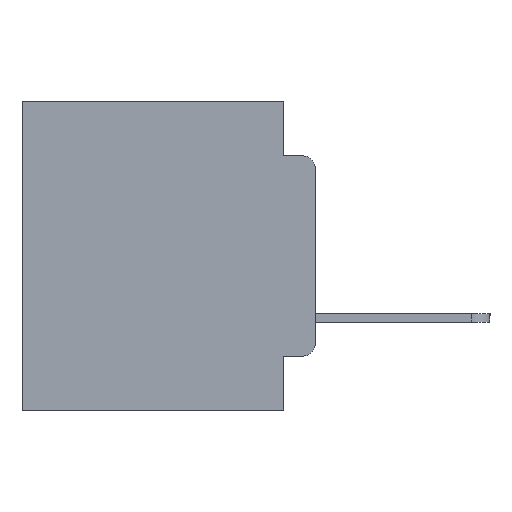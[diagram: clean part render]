
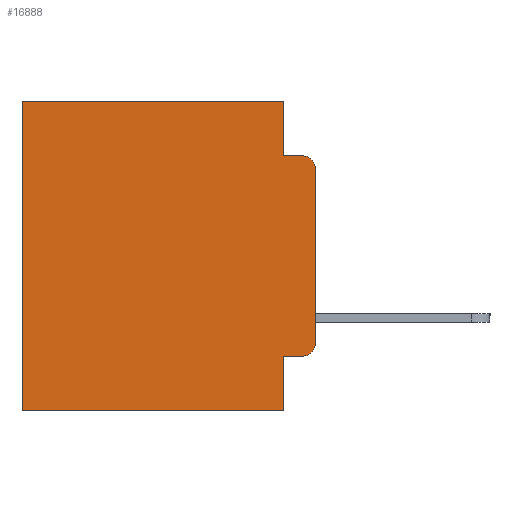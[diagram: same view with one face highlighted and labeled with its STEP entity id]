
A CAD part, left-side view. The second image highlights one B-rep face of the part: STEP entity #16888.
In plain terms, the highlighted planar face has unit normal (-1, 0, 0).
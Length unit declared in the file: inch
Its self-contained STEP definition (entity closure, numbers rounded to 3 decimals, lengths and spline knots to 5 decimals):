
#23 = CARTESIAN_POINT ( 'NONE',  ( 0.298, 0.02, -0.1085 ) ) ;
#478 = VERTEX_POINT ( 'NONE', #4145 ) ;
#646 = CARTESIAN_POINT ( 'NONE',  ( 0.298, 0.051, -0.4115 ) ) ;
#1078 = DIRECTION ( 'NONE',  ( 0., 1., 0. ) ) ;
#1101 = DIRECTION ( 'NONE',  ( 0., 0., -1. ) ) ;
#1195 = EDGE_CURVE ( 'NONE', #14143, #478, #6754, .T. ) ;
#1214 = DIRECTION ( 'NONE',  ( -1., 0., 0. ) ) ;
#1450 = ORIENTED_EDGE ( 'NONE', *, *, #19248, .T. ) ;
#1597 = VERTEX_POINT ( 'NONE', #25536 ) ;
#1932 = CARTESIAN_POINT ( 'NONE',  ( 0.298, 0.051, -0.0885 ) ) ;
#2301 = PLANE ( 'NONE',  #19564 ) ;
#2484 = ORIENTED_EDGE ( 'NONE', *, *, #11414, .F. ) ;
#2971 = CARTESIAN_POINT ( 'NONE',  ( 0.298, 0.051, 0. ) ) ;
#3621 = VECTOR ( 'NONE', #20673, 39.37008 ) ;
#3719 = DIRECTION ( 'NONE',  ( 0., 0., -1. ) ) ;
#3796 = VECTOR ( 'NONE', #16145, 39.37008 ) ;
#4145 = CARTESIAN_POINT ( 'NONE',  ( 0.298, 0.02, -0.0885 ) ) ;
#4372 = EDGE_CURVE ( 'NONE', #14143, #24599, #4515, .T. ) ;
#4515 = LINE ( 'NONE', #25335, #20131 ) ;
#4673 = DIRECTION ( 'NONE',  ( 1., 0., 0. ) ) ;
#5007 = ORIENTED_EDGE ( 'NONE', *, *, #18590, .T. ) ;
#5626 = CARTESIAN_POINT ( 'NONE',  ( 0.298, 0.02, -0.4115 ) ) ;
#5757 = CARTESIAN_POINT ( 'NONE',  ( 0.298, 0.473, -0.5 ) ) ;
#6733 = VERTEX_POINT ( 'NONE', #11327 ) ;
#6754 = CIRCLE ( 'NONE', #20855, 0.02 ) ;
#7648 = DIRECTION ( 'NONE',  ( 0., 0., -1. ) ) ;
#7966 = CARTESIAN_POINT ( 'NONE',  ( 0.298, 0.02, -0.3915 ) ) ;
#8065 = CARTESIAN_POINT ( 'NONE',  ( 0.298, 0.473, 0. ) ) ;
#8209 = CARTESIAN_POINT ( 'NONE',  ( 0.298, 0.051, -0.0885 ) ) ;
#8660 = EDGE_LOOP ( 'NONE', ( #14326, #27392, #18830, #18717, #5007, #10817, #2484, #20931, #25911, #1450 ) ) ;
#9316 = CARTESIAN_POINT ( 'NONE',  ( 0.298, 0., -0.1085 ) ) ;
#9492 = LINE ( 'NONE', #16740, #20397 ) ;
#9797 = VERTEX_POINT ( 'NONE', #1932 ) ;
#9856 = CARTESIAN_POINT ( 'NONE',  ( 0.298, 0.051, -0.4115 ) ) ;
#10283 = DIRECTION ( 'NONE',  ( 0., 0., -1. ) ) ;
#10361 = VECTOR ( 'NONE', #1078, 39.37008 ) ;
#10817 = ORIENTED_EDGE ( 'NONE', *, *, #24540, .T. ) ;
#11327 = CARTESIAN_POINT ( 'NONE',  ( 0.298, 0.051, 0. ) ) ;
#11414 = EDGE_CURVE ( 'NONE', #1597, #17943, #16556, .T. ) ;
#11442 = AXIS2_PLACEMENT_3D ( 'NONE', #7966, #22466, #10283 ) ;
#11803 = LINE ( 'NONE', #14693, #16550 ) ;
#14119 = FACE_OUTER_BOUND ( 'NONE', #8660, .T. ) ;
#14143 = VERTEX_POINT ( 'NONE', #9316 ) ;
#14173 = LINE ( 'NONE', #646, #3796 ) ;
#14326 = ORIENTED_EDGE ( 'NONE', *, *, #4372, .F. ) ;
#14484 = VERTEX_POINT ( 'NONE', #8065 ) ;
#14693 = CARTESIAN_POINT ( 'NONE',  ( 0.298, 0.473, 0. ) ) ;
#15055 = LINE ( 'NONE', #2971, #20416 ) ;
#15730 = CARTESIAN_POINT ( 'NONE',  ( 0.298, 0., -0.5 ) ) ;
#16145 = DIRECTION ( 'NONE',  ( 0., -1., 0. ) ) ;
#16550 = VECTOR ( 'NONE', #3719, 39.37008 ) ;
#16556 = LINE ( 'NONE', #15730, #19122 ) ;
#16740 = CARTESIAN_POINT ( 'NONE',  ( 0.298, 0.051, 0. ) ) ;
#16888 = ADVANCED_FACE ( 'NONE', ( #14119 ), #2301, .F. ) ;
#17550 = CARTESIAN_POINT ( 'NONE',  ( 0.298, 0., 0. ) ) ;
#17766 = VERTEX_POINT ( 'NONE', #9856 ) ;
#17943 = VERTEX_POINT ( 'NONE', #5757 ) ;
#18559 = CARTESIAN_POINT ( 'NONE',  ( 0.298, 0., 0. ) ) ;
#18590 = EDGE_CURVE ( 'NONE', #6733, #14484, #21212, .T. ) ;
#18717 = ORIENTED_EDGE ( 'NONE', *, *, #25830, .F. ) ;
#18800 = DIRECTION ( 'NONE',  ( 0., 0., -1. ) ) ;
#18830 = ORIENTED_EDGE ( 'NONE', *, *, #27117, .F. ) ;
#19122 = VECTOR ( 'NONE', #25737, 39.37008 ) ;
#19248 = EDGE_CURVE ( 'NONE', #23685, #24599, #19906, .T. ) ;
#19564 = AXIS2_PLACEMENT_3D ( 'NONE', #17550, #4673, #19574 ) ;
#19574 = DIRECTION ( 'NONE',  ( 0., 0., -1. ) ) ;
#19906 = CIRCLE ( 'NONE', #11442, 0.02 ) ;
#20131 = VECTOR ( 'NONE', #27250, 39.37008 ) ;
#20397 = VECTOR ( 'NONE', #18800, 39.37008 ) ;
#20416 = VECTOR ( 'NONE', #7648, 39.37008 ) ;
#20565 = EDGE_CURVE ( 'NONE', #17766, #23685, #14173, .T. ) ;
#20673 = DIRECTION ( 'NONE',  ( 0., -1., 0. ) ) ;
#20855 = AXIS2_PLACEMENT_3D ( 'NONE', #23, #1214, #1101 ) ;
#20873 = CARTESIAN_POINT ( 'NONE',  ( 0.298, 0., -0.3915 ) ) ;
#20931 = ORIENTED_EDGE ( 'NONE', *, *, #21934, .F. ) ;
#21212 = LINE ( 'NONE', #18559, #10361 ) ;
#21934 = EDGE_CURVE ( 'NONE', #17766, #1597, #15055, .T. ) ;
#22466 = DIRECTION ( 'NONE',  ( -1., 0., 0. ) ) ;
#23685 = VERTEX_POINT ( 'NONE', #5626 ) ;
#24540 = EDGE_CURVE ( 'NONE', #14484, #17943, #11803, .T. ) ;
#24599 = VERTEX_POINT ( 'NONE', #20873 ) ;
#25274 = LINE ( 'NONE', #8209, #3621 ) ;
#25335 = CARTESIAN_POINT ( 'NONE',  ( 0.298, 0., 0. ) ) ;
#25536 = CARTESIAN_POINT ( 'NONE',  ( 0.298, 0.051, -0.5 ) ) ;
#25737 = DIRECTION ( 'NONE',  ( 0., 1., 0. ) ) ;
#25830 = EDGE_CURVE ( 'NONE', #6733, #9797, #9492, .T. ) ;
#25911 = ORIENTED_EDGE ( 'NONE', *, *, #20565, .T. ) ;
#27117 = EDGE_CURVE ( 'NONE', #9797, #478, #25274, .T. ) ;
#27250 = DIRECTION ( 'NONE',  ( 0., 0., -1. ) ) ;
#27392 = ORIENTED_EDGE ( 'NONE', *, *, #1195, .T. ) ;
